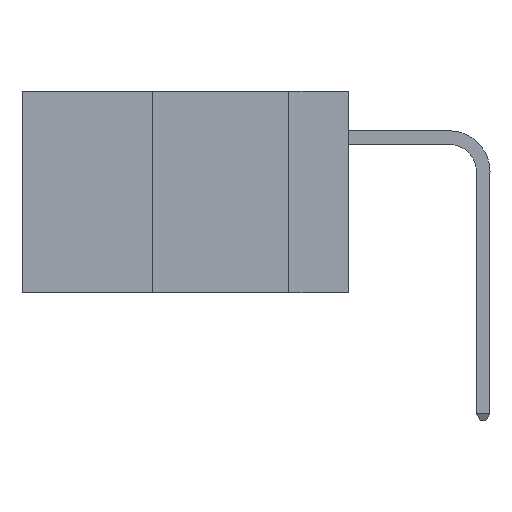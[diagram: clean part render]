
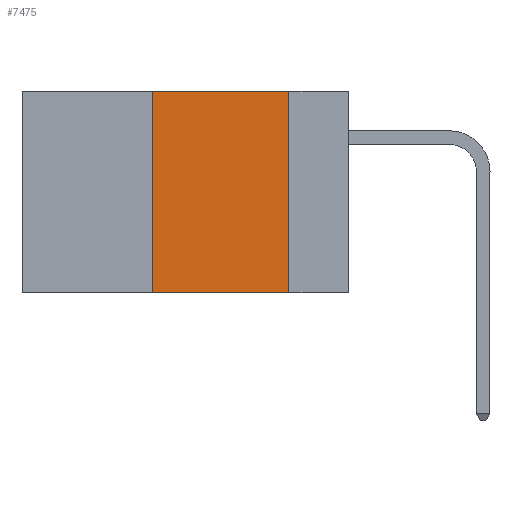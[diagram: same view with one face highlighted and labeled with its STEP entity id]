
A CAD part, left-side view. The second image highlights one B-rep face of the part: STEP entity #7475.
In plain terms, the highlighted planar face has unit normal (-1, 0, 0).
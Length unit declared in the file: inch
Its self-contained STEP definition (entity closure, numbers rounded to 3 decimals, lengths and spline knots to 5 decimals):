
#535 = DIRECTION ( 'NONE',  ( 0., -1., 0. ) ) ;
#893 = CARTESIAN_POINT ( 'NONE',  ( 0., 0.36, 0. ) ) ;
#968 = LINE ( 'NONE', #893, #11607 ) ;
#1118 = CARTESIAN_POINT ( 'NONE',  ( 0., 0.11, -0.37 ) ) ;
#1536 = VECTOR ( 'NONE', #9573, 39.37008 ) ;
#1898 = LINE ( 'NONE', #11515, #7328 ) ;
#2645 = CARTESIAN_POINT ( 'NONE',  ( 0., 0.36, -0.37 ) ) ;
#3121 = EDGE_CURVE ( 'NONE', #20324, #4614, #20289, .T. ) ;
#4389 = ORIENTED_EDGE ( 'NONE', *, *, #7460, .F. ) ;
#4614 = VERTEX_POINT ( 'NONE', #6688 ) ;
#5824 = VECTOR ( 'NONE', #535, 39.37008 ) ;
#6688 = CARTESIAN_POINT ( 'NONE',  ( 0., 0.11, 0. ) ) ;
#7039 = ORIENTED_EDGE ( 'NONE', *, *, #11567, .T. ) ;
#7328 = VECTOR ( 'NONE', #11666, 39.37008 ) ;
#7460 = EDGE_CURVE ( 'NONE', #4614, #13461, #1898, .T. ) ;
#7475 = ADVANCED_FACE ( 'NONE', ( #21191 ), #21963, .F. ) ;
#7936 = DIRECTION ( 'NONE',  ( 0., 0., -1. ) ) ;
#9573 = DIRECTION ( 'NONE',  ( 0., -1., 0. ) ) ;
#9615 = AXIS2_PLACEMENT_3D ( 'NONE', #9888, #22112, #7936 ) ;
#9888 = CARTESIAN_POINT ( 'NONE',  ( 0., 0.6, 0. ) ) ;
#11515 = CARTESIAN_POINT ( 'NONE',  ( 0., 0.11, 0. ) ) ;
#11567 = EDGE_CURVE ( 'NONE', #16912, #13461, #15088, .T. ) ;
#11607 = VECTOR ( 'NONE', #13281, 39.37008 ) ;
#11666 = DIRECTION ( 'NONE',  ( 0., 0., -1. ) ) ;
#12355 = ORIENTED_EDGE ( 'NONE', *, *, #3121, .F. ) ;
#12870 = CARTESIAN_POINT ( 'NONE',  ( 0., 0.6, 0. ) ) ;
#13281 = DIRECTION ( 'NONE',  ( 0., 0., 1. ) ) ;
#13356 = CARTESIAN_POINT ( 'NONE',  ( 0., 0.6, -0.37 ) ) ;
#13461 = VERTEX_POINT ( 'NONE', #1118 ) ;
#14475 = CARTESIAN_POINT ( 'NONE',  ( 0., 0.36, 0. ) ) ;
#15088 = LINE ( 'NONE', #13356, #5824 ) ;
#15610 = ORIENTED_EDGE ( 'NONE', *, *, #19917, .F. ) ;
#16667 = EDGE_LOOP ( 'NONE', ( #4389, #12355, #15610, #7039 ) ) ;
#16912 = VERTEX_POINT ( 'NONE', #2645 ) ;
#19917 = EDGE_CURVE ( 'NONE', #16912, #20324, #968, .T. ) ;
#20289 = LINE ( 'NONE', #12870, #1536 ) ;
#20324 = VERTEX_POINT ( 'NONE', #14475 ) ;
#21191 = FACE_OUTER_BOUND ( 'NONE', #16667, .T. ) ;
#21963 = PLANE ( 'NONE',  #9615 ) ;
#22112 = DIRECTION ( 'NONE',  ( 1., 0., 0. ) ) ;
